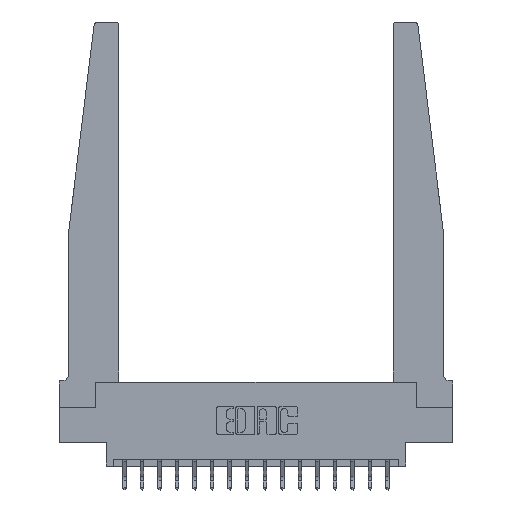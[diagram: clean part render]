
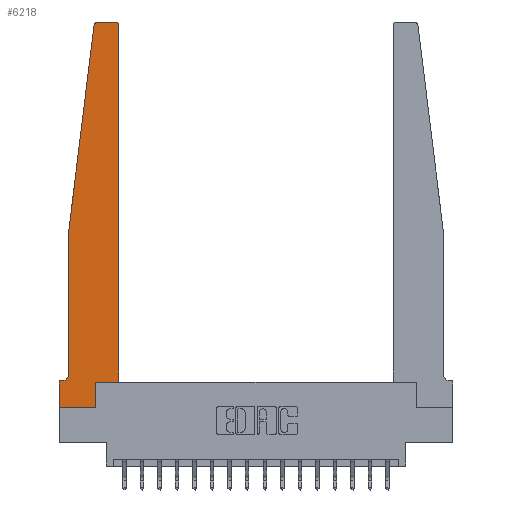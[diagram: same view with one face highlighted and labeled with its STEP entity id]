
A CAD part, top view. The second image highlights one B-rep face of the part: STEP entity #6218.
In plain terms, the highlighted planar face has unit normal (0, 0, 1).
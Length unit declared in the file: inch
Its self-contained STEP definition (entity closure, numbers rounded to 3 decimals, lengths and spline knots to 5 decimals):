
#290 = VECTOR ( 'NONE', #19262, 39.37008 ) ;
#544 = LINE ( 'NONE', #11196, #2868 ) ;
#1014 = CARTESIAN_POINT ( 'NONE',  ( 0.425, 0.18, 0.37 ) ) ;
#1247 = EDGE_CURVE ( 'NONE', #5258, #7390, #12074, .T. ) ;
#1318 = CARTESIAN_POINT ( 'NONE',  ( 0.24675, 2.72367, 0.37 ) ) ;
#1479 = ORIENTED_EDGE ( 'NONE', *, *, #1247, .T. ) ;
#1768 = CARTESIAN_POINT ( 'NONE',  ( 0.2605, 0.18, 0.37 ) ) ;
#1912 = FACE_OUTER_BOUND ( 'NONE', #16201, .T. ) ;
#2171 = CARTESIAN_POINT ( 'NONE',  ( 0.065, 1.25, 0.37 ) ) ;
#2545 = CARTESIAN_POINT ( 'NONE',  ( 0.2605, 0., 0.37 ) ) ;
#2687 = ORIENTED_EDGE ( 'NONE', *, *, #8024, .T. ) ;
#2739 = CARTESIAN_POINT ( 'NONE',  ( 0.425, 0.18, 0.37 ) ) ;
#2868 = VECTOR ( 'NONE', #5393, 39.37008 ) ;
#3056 = VERTEX_POINT ( 'NONE', #13493 ) ;
#3172 = VERTEX_POINT ( 'NONE', #11190 ) ;
#3344 = CIRCLE ( 'NONE', #10895, 0.05 ) ;
#3401 = CARTESIAN_POINT ( 'NONE',  ( 0.065, 0.2375, 0.37 ) ) ;
#3484 = DIRECTION ( 'NONE',  ( -1., 0., 0. ) ) ;
#3650 = DIRECTION ( 'NONE',  ( 1., 0., 0. ) ) ;
#3720 = DIRECTION ( 'NONE',  ( -1., 0., 0. ) ) ;
#3842 = ORIENTED_EDGE ( 'NONE', *, *, #10413, .T. ) ;
#4144 = LINE ( 'NONE', #7509, #16058 ) ;
#4168 = VECTOR ( 'NONE', #4787, 39.37008 ) ;
#4372 = LINE ( 'NONE', #4568, #290 ) ;
#4568 = CARTESIAN_POINT ( 'NONE',  ( 0.065, 1.25, 0.37 ) ) ;
#4787 = DIRECTION ( 'NONE',  ( -1., 0., 0. ) ) ;
#4794 = CARTESIAN_POINT ( 'NONE',  ( 0., 0.1875, 0.37 ) ) ;
#4887 = DIRECTION ( 'NONE',  ( 1., 0., 0. ) ) ;
#5164 = ORIENTED_EDGE ( 'NONE', *, *, #17938, .T. ) ;
#5258 = VERTEX_POINT ( 'NONE', #15658 ) ;
#5393 = DIRECTION ( 'NONE',  ( 0., 1., 0. ) ) ;
#5922 = AXIS2_PLACEMENT_3D ( 'NONE', #17288, #6667, #8231 ) ;
#6129 = EDGE_CURVE ( 'NONE', #16188, #17649, #18427, .T. ) ;
#6218 = ADVANCED_FACE ( 'NONE', ( #1912 ), #10893, .T. ) ;
#6667 = DIRECTION ( 'NONE',  ( 0., 0., 1. ) ) ;
#6978 = VERTEX_POINT ( 'NONE', #1768 ) ;
#7229 = VERTEX_POINT ( 'NONE', #2739 ) ;
#7275 = VERTEX_POINT ( 'NONE', #2545 ) ;
#7390 = VERTEX_POINT ( 'NONE', #4794 ) ;
#7394 = VECTOR ( 'NONE', #3650, 39.37008 ) ;
#7509 = CARTESIAN_POINT ( 'NONE',  ( 0., 0., 0.37 ) ) ;
#7684 = EDGE_CURVE ( 'NONE', #3056, #11775, #4372, .T. ) ;
#7935 = DIRECTION ( 'NONE',  ( 1., 0., 0. ) ) ;
#8024 = EDGE_CURVE ( 'NONE', #10425, #3056, #15666, .T. ) ;
#8231 = DIRECTION ( 'NONE',  ( 1., 0., 0. ) ) ;
#8726 = EDGE_CURVE ( 'NONE', #11002, #7275, #11833, .T. ) ;
#8820 = VECTOR ( 'NONE', #3484, 39.37008 ) ;
#8821 = ORIENTED_EDGE ( 'NONE', *, *, #10231, .T. ) ;
#8888 = CARTESIAN_POINT ( 'NONE',  ( 0., 0., 0.37 ) ) ;
#8991 = AXIS2_PLACEMENT_3D ( 'NONE', #16897, #9406, #7935 ) ;
#9121 = ORIENTED_EDGE ( 'NONE', *, *, #7684, .T. ) ;
#9403 = LINE ( 'NONE', #10794, #4168 ) ;
#9406 = DIRECTION ( 'NONE',  ( 0., 0., 1. ) ) ;
#9629 = EDGE_CURVE ( 'NONE', #7390, #11002, #4144, .T. ) ;
#10210 = CARTESIAN_POINT ( 'NONE',  ( 0.425, 2.72, 0.37 ) ) ;
#10231 = EDGE_CURVE ( 'NONE', #7275, #6978, #544, .T. ) ;
#10251 = ORIENTED_EDGE ( 'NONE', *, *, #11784, .T. ) ;
#10265 = DIRECTION ( 'NONE',  ( 0., -1., 0. ) ) ;
#10413 = EDGE_CURVE ( 'NONE', #7229, #16188, #19371, .T. ) ;
#10425 = VERTEX_POINT ( 'NONE', #1318 ) ;
#10794 = CARTESIAN_POINT ( 'NONE',  ( 0.25, 2.75, 0.37 ) ) ;
#10893 = PLANE ( 'NONE',  #8991 ) ;
#10895 = AXIS2_PLACEMENT_3D ( 'NONE', #18603, #11206, #3720 ) ;
#11002 = VERTEX_POINT ( 'NONE', #8888 ) ;
#11056 = VECTOR ( 'NONE', #11347, 39.37008 ) ;
#11190 = CARTESIAN_POINT ( 'NONE',  ( 0.27653, 2.75, 0.37 ) ) ;
#11196 = CARTESIAN_POINT ( 'NONE',  ( 0.2605, 0.18, 0.37 ) ) ;
#11206 = DIRECTION ( 'NONE',  ( 0., 0., -1. ) ) ;
#11347 = DIRECTION ( 'NONE',  ( -0.122, -0.992, 0. ) ) ;
#11548 = ORIENTED_EDGE ( 'NONE', *, *, #8726, .T. ) ;
#11693 = VECTOR ( 'NONE', #19215, 39.37008 ) ;
#11775 = VERTEX_POINT ( 'NONE', #3401 ) ;
#11784 = EDGE_CURVE ( 'NONE', #17649, #3172, #9403, .T. ) ;
#11809 = ORIENTED_EDGE ( 'NONE', *, *, #6129, .T. ) ;
#11833 = LINE ( 'NONE', #13211, #11693 ) ;
#12074 = LINE ( 'NONE', #18072, #8820 ) ;
#12484 = DIRECTION ( 'NONE',  ( 0., 0., 1. ) ) ;
#12546 = LINE ( 'NONE', #17135, #7394 ) ;
#12823 = ORIENTED_EDGE ( 'NONE', *, *, #14104, .T. ) ;
#13211 = CARTESIAN_POINT ( 'NONE',  ( 0., 0., 0.37 ) ) ;
#13493 = CARTESIAN_POINT ( 'NONE',  ( 0.065, 1.25, 0.37 ) ) ;
#13587 = VECTOR ( 'NONE', #16010, 39.37008 ) ;
#14104 = EDGE_CURVE ( 'NONE', #6978, #7229, #12546, .T. ) ;
#15599 = ORIENTED_EDGE ( 'NONE', *, *, #9629, .T. ) ;
#15634 = CIRCLE ( 'NONE', #5922, 0.03 ) ;
#15658 = CARTESIAN_POINT ( 'NONE',  ( 0.015, 0.1875, 0.37 ) ) ;
#15666 = LINE ( 'NONE', #2171, #11056 ) ;
#16010 = DIRECTION ( 'NONE',  ( 0., 1., 0. ) ) ;
#16058 = VECTOR ( 'NONE', #10265, 39.37008 ) ;
#16188 = VERTEX_POINT ( 'NONE', #10210 ) ;
#16201 = EDGE_LOOP ( 'NONE', ( #10251, #18111, #2687, #9121, #5164, #1479, #15599, #11548, #8821, #12823, #3842, #11809 ) ) ;
#16897 = CARTESIAN_POINT ( 'NONE',  ( 0., 0.1875, 0.37 ) ) ;
#17135 = CARTESIAN_POINT ( 'NONE',  ( 0.425, 0.18, 0.37 ) ) ;
#17288 = CARTESIAN_POINT ( 'NONE',  ( 0.27653, 2.72, 0.37 ) ) ;
#17649 = VERTEX_POINT ( 'NONE', #18086 ) ;
#17938 = EDGE_CURVE ( 'NONE', #11775, #5258, #3344, .T. ) ;
#18072 = CARTESIAN_POINT ( 'NONE',  ( 0.065, 0.1875, 0.37 ) ) ;
#18086 = CARTESIAN_POINT ( 'NONE',  ( 0.395, 2.75, 0.37 ) ) ;
#18111 = ORIENTED_EDGE ( 'NONE', *, *, #19399, .T. ) ;
#18188 = CARTESIAN_POINT ( 'NONE',  ( 0.395, 2.72, 0.37 ) ) ;
#18427 = CIRCLE ( 'NONE', #19040, 0.03 ) ;
#18603 = CARTESIAN_POINT ( 'NONE',  ( 0.015, 0.2375, 0.37 ) ) ;
#19040 = AXIS2_PLACEMENT_3D ( 'NONE', #18188, #12484, #4887 ) ;
#19215 = DIRECTION ( 'NONE',  ( 1., 0., 0. ) ) ;
#19262 = DIRECTION ( 'NONE',  ( 0., -1., 0. ) ) ;
#19371 = LINE ( 'NONE', #1014, #13587 ) ;
#19399 = EDGE_CURVE ( 'NONE', #3172, #10425, #15634, .T. ) ;
